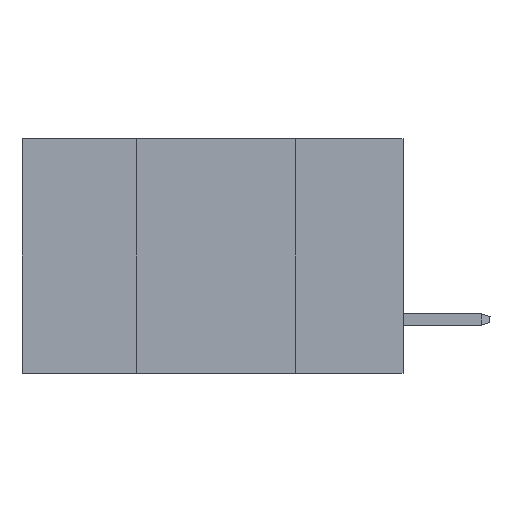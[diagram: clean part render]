
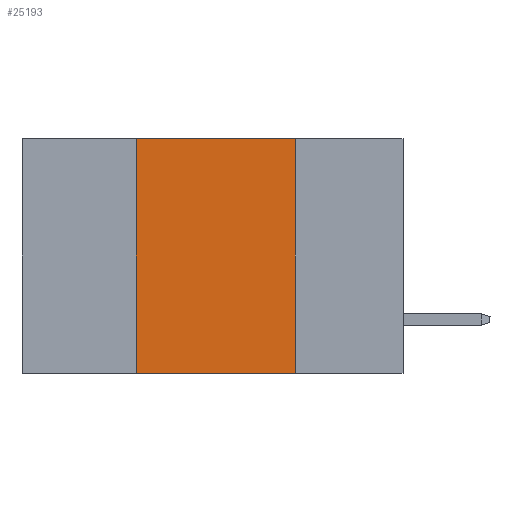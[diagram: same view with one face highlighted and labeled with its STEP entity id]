
A CAD part, left-side view. The second image highlights one B-rep face of the part: STEP entity #25193.
In plain terms, the highlighted planar face has unit normal (-1, 0, 0).
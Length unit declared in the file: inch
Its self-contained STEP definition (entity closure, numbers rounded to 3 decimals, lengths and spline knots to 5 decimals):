
#1046 = CARTESIAN_POINT ( 'NONE',  ( 0., 0.6, 0. ) ) ;
#3589 = DIRECTION ( 'NONE',  ( 0., 0., 1. ) ) ;
#5227 = EDGE_CURVE ( 'NONE', #25166, #34397, #21783, .T. ) ;
#5535 = VERTEX_POINT ( 'NONE', #22895 ) ;
#6512 = ORIENTED_EDGE ( 'NONE', *, *, #20407, .F. ) ;
#6602 = CARTESIAN_POINT ( 'NONE',  ( 0., 0.42, 0. ) ) ;
#8432 = AXIS2_PLACEMENT_3D ( 'NONE', #1046, #25237, #19285 ) ;
#9935 = ORIENTED_EDGE ( 'NONE', *, *, #5227, .F. ) ;
#10356 = PLANE ( 'NONE',  #8432 ) ;
#11483 = EDGE_CURVE ( 'NONE', #34397, #14884, #16453, .T. ) ;
#11889 = DIRECTION ( 'NONE',  ( 0., -1., 0. ) ) ;
#13584 = LINE ( 'NONE', #31428, #18623 ) ;
#14884 = VERTEX_POINT ( 'NONE', #25557 ) ;
#16453 = LINE ( 'NONE', #25192, #30704 ) ;
#17691 = ORIENTED_EDGE ( 'NONE', *, *, #26902, .T. ) ;
#18623 = VECTOR ( 'NONE', #25682, 39.37008 ) ;
#19285 = DIRECTION ( 'NONE',  ( 0., 0., -1. ) ) ;
#20407 = EDGE_CURVE ( 'NONE', #5535, #25166, #36685, .T. ) ;
#21011 = VECTOR ( 'NONE', #3589, 39.37008 ) ;
#21079 = VECTOR ( 'NONE', #11889, 39.37008 ) ;
#21783 = LINE ( 'NONE', #26976, #21079 ) ;
#22665 = ORIENTED_EDGE ( 'NONE', *, *, #11483, .F. ) ;
#22895 = CARTESIAN_POINT ( 'NONE',  ( 0., 0.42, -0.37 ) ) ;
#25166 = VERTEX_POINT ( 'NONE', #6602 ) ;
#25192 = CARTESIAN_POINT ( 'NONE',  ( 0., 0.17, 0. ) ) ;
#25193 = ADVANCED_FACE ( 'NONE', ( #37516 ), #10356, .F. ) ;
#25237 = DIRECTION ( 'NONE',  ( 1., 0., 0. ) ) ;
#25463 = CARTESIAN_POINT ( 'NONE',  ( 0., 0.17, 0. ) ) ;
#25557 = CARTESIAN_POINT ( 'NONE',  ( 0., 0.17, -0.37 ) ) ;
#25682 = DIRECTION ( 'NONE',  ( 0., -1., 0. ) ) ;
#26902 = EDGE_CURVE ( 'NONE', #5535, #14884, #13584, .T. ) ;
#26976 = CARTESIAN_POINT ( 'NONE',  ( 0., 0.6, 0. ) ) ;
#28563 = DIRECTION ( 'NONE',  ( 0., 0., -1. ) ) ;
#30405 = EDGE_LOOP ( 'NONE', ( #22665, #9935, #6512, #17691 ) ) ;
#30704 = VECTOR ( 'NONE', #28563, 39.37008 ) ;
#30744 = CARTESIAN_POINT ( 'NONE',  ( 0., 0.42, 0. ) ) ;
#31428 = CARTESIAN_POINT ( 'NONE',  ( 0., 0.6, -0.37 ) ) ;
#34397 = VERTEX_POINT ( 'NONE', #25463 ) ;
#36685 = LINE ( 'NONE', #30744, #21011 ) ;
#37516 = FACE_OUTER_BOUND ( 'NONE', #30405, .T. ) ;
